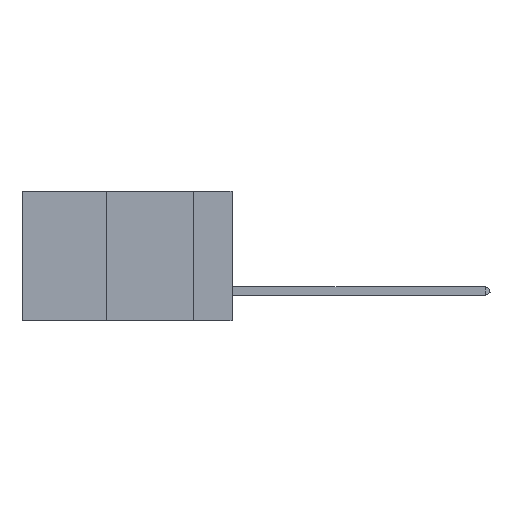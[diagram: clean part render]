
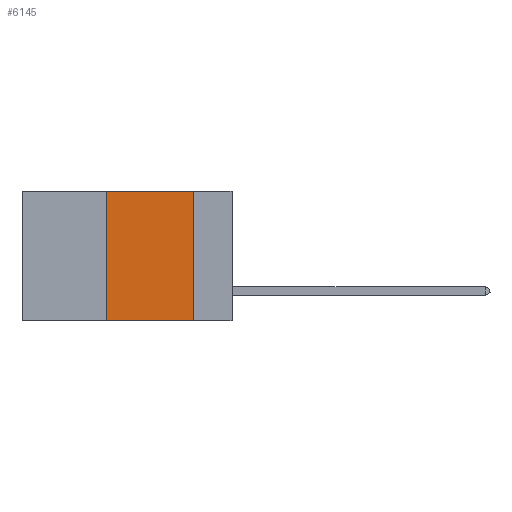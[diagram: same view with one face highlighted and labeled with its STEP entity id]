
A CAD part, left-side view. The second image highlights one B-rep face of the part: STEP entity #6145.
In plain terms, the highlighted planar face has unit normal (-1, 0, 0).
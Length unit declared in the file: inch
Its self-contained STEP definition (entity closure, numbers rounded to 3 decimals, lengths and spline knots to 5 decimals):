
#333 = VECTOR ( 'NONE', #5395, 39.37008 ) ;
#1219 = PLANE ( 'NONE',  #3286 ) ;
#2037 = EDGE_CURVE ( 'NONE', #6402, #14653, #14419, .T. ) ;
#2786 = ORIENTED_EDGE ( 'NONE', *, *, #9446, .F. ) ;
#3286 = AXIS2_PLACEMENT_3D ( 'NONE', #9026, #9091, #10706 ) ;
#4125 = DIRECTION ( 'NONE',  ( 0., 0., 1. ) ) ;
#4197 = FACE_OUTER_BOUND ( 'NONE', #19165, .T. ) ;
#4624 = LINE ( 'NONE', #8452, #333 ) ;
#4849 = VERTEX_POINT ( 'NONE', #13017 ) ;
#5395 = DIRECTION ( 'NONE',  ( 0., -1., 0. ) ) ;
#6022 = ORIENTED_EDGE ( 'NONE', *, *, #14312, .T. ) ;
#6145 = ADVANCED_FACE ( 'NONE', ( #4197 ), #1219, .F. ) ;
#6402 = VERTEX_POINT ( 'NONE', #11092 ) ;
#7631 = LINE ( 'NONE', #8330, #9555 ) ;
#7926 = ORIENTED_EDGE ( 'NONE', *, *, #8795, .F. ) ;
#8330 = CARTESIAN_POINT ( 'NONE',  ( 0., 0.6, -0.37 ) ) ;
#8452 = CARTESIAN_POINT ( 'NONE',  ( 0., 0.6, 0. ) ) ;
#8795 = EDGE_CURVE ( 'NONE', #10961, #6402, #4624, .T. ) ;
#8939 = DIRECTION ( 'NONE',  ( 0., 0., -1. ) ) ;
#9010 = CARTESIAN_POINT ( 'NONE',  ( 0., 0.11, 0. ) ) ;
#9026 = CARTESIAN_POINT ( 'NONE',  ( 0., 0.6, 0. ) ) ;
#9091 = DIRECTION ( 'NONE',  ( 1., 0., 0. ) ) ;
#9446 = EDGE_CURVE ( 'NONE', #4849, #10961, #13686, .T. ) ;
#9555 = VECTOR ( 'NONE', #11488, 39.37008 ) ;
#10434 = CARTESIAN_POINT ( 'NONE',  ( 0., 0.11, -0.37 ) ) ;
#10706 = DIRECTION ( 'NONE',  ( 0., 0., -1. ) ) ;
#10961 = VERTEX_POINT ( 'NONE', #19123 ) ;
#11092 = CARTESIAN_POINT ( 'NONE',  ( 0., 0.11, 0. ) ) ;
#11467 = VECTOR ( 'NONE', #8939, 39.37008 ) ;
#11488 = DIRECTION ( 'NONE',  ( 0., -1., 0. ) ) ;
#11661 = CARTESIAN_POINT ( 'NONE',  ( 0., 0.36, 0. ) ) ;
#13017 = CARTESIAN_POINT ( 'NONE',  ( 0., 0.36, -0.37 ) ) ;
#13686 = LINE ( 'NONE', #11661, #18561 ) ;
#14312 = EDGE_CURVE ( 'NONE', #4849, #14653, #7631, .T. ) ;
#14419 = LINE ( 'NONE', #9010, #11467 ) ;
#14653 = VERTEX_POINT ( 'NONE', #10434 ) ;
#17217 = ORIENTED_EDGE ( 'NONE', *, *, #2037, .F. ) ;
#18561 = VECTOR ( 'NONE', #4125, 39.37008 ) ;
#19123 = CARTESIAN_POINT ( 'NONE',  ( 0., 0.36, 0. ) ) ;
#19165 = EDGE_LOOP ( 'NONE', ( #17217, #7926, #2786, #6022 ) ) ;
